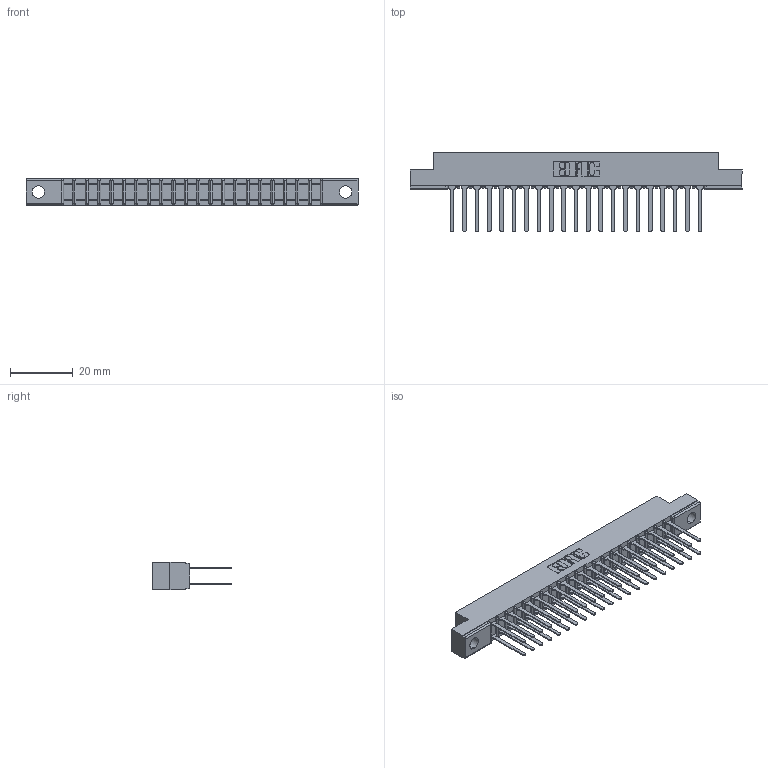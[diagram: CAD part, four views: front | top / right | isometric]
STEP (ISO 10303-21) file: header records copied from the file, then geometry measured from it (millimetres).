
FILE_DESCRIPTION (( 'STEP AP203' ), '1' );
FILE_NAME ('307-042-542-204.STEP', '2019-09-06T06:39:49', ( '' ), ( '' ), 'SwSTEP 2.0', 'SolidWorks 2016', '' );
FILE_SCHEMA (( 'CONFIG_CONTROL_DESIGN' ));
Length unit declared in the file: inch
Products named in the file (3): 307 Part_.156 Dia Mounting Holes; 307-042-542-204; 307-290-001_542
Assembly tree (43 placements, depth 2):
  307-042-542-204
    307 Part_.156 Dia Mounting Holes
    307-290-001_542  x42
Bounding box: 106.22 x 25.43 x 8.71 mm (x, y, z)
Volume: 7002.7 mm3; surface area: 13098.3 mm2
Topology: 43 solids, 43 shells, 2086 faces, 5819 edges, 3762 vertices
Faces by surface type: plane 1386, cylinder 656, sphere 44
Entity records: 21650 total; most frequent: CARTESIAN_POINT 3551, ORIENTED_EDGE 3514, DIRECTION 3479, EDGE_CURVE 1757, VECTOR 1347, LINE 1347, VERTEX_POINT 1138, AXIS2_PLACEMENT_3D 1066
